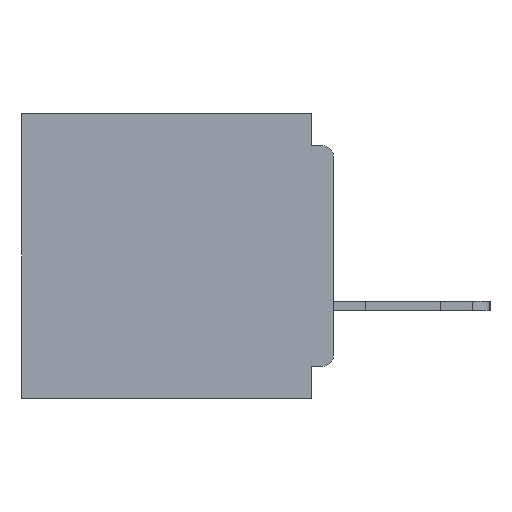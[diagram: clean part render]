
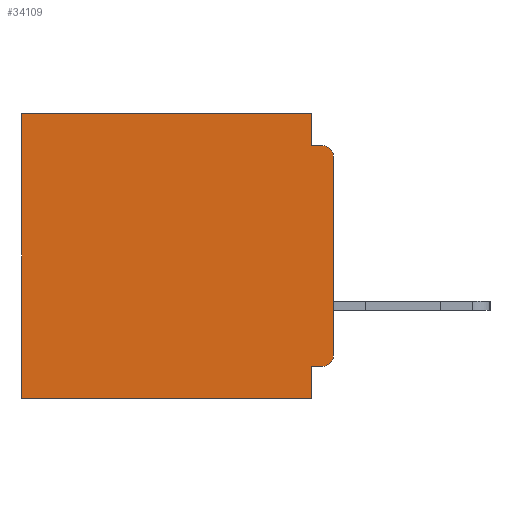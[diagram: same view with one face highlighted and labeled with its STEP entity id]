
A CAD part, left-side view. The second image highlights one B-rep face of the part: STEP entity #34109.
In plain terms, the highlighted planar face has unit normal (-1, 0, 0).
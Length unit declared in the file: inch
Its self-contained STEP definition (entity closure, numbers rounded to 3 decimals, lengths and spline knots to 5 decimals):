
#508 = EDGE_LOOP ( 'NONE', ( #7604, #32701, #13063, #24815, #25394, #37105, #4179, #37846, #33562, #59256 ) ) ;
#1082 = CARTESIAN_POINT ( 'NONE',  ( 0.3, 0., -0.4 ) ) ;
#1469 = VERTEX_POINT ( 'NONE', #15467 ) ;
#1531 = LINE ( 'NONE', #14332, #25078 ) ;
#3493 = CARTESIAN_POINT ( 'NONE',  ( 0.3, 0.015, -0.355 ) ) ;
#4179 = ORIENTED_EDGE ( 'NONE', *, *, #61066, .F. ) ;
#4317 = LINE ( 'NONE', #37463, #62940 ) ;
#5022 = DIRECTION ( 'NONE',  ( 0., 0., -1. ) ) ;
#5680 = EDGE_CURVE ( 'NONE', #12072, #39543, #38894, .T. ) ;
#5737 = CARTESIAN_POINT ( 'NONE',  ( 0.3, 0.031, -0.4 ) ) ;
#6200 = DIRECTION ( 'NONE',  ( 0., 0., -1. ) ) ;
#7165 = FACE_OUTER_BOUND ( 'NONE', #508, .T. ) ;
#7604 = ORIENTED_EDGE ( 'NONE', *, *, #63134, .F. ) ;
#8185 = LINE ( 'NONE', #50016, #62896 ) ;
#9714 = DIRECTION ( 'NONE',  ( -1., 0., 0. ) ) ;
#9831 = CARTESIAN_POINT ( 'NONE',  ( 0.3, 0., 0. ) ) ;
#12072 = VERTEX_POINT ( 'NONE', #62257 ) ;
#13063 = ORIENTED_EDGE ( 'NONE', *, *, #31377, .F. ) ;
#14090 = DIRECTION ( 'NONE',  ( 0., 0., -1. ) ) ;
#14332 = CARTESIAN_POINT ( 'NONE',  ( 0.3, 0., -0.4 ) ) ;
#14398 = AXIS2_PLACEMENT_3D ( 'NONE', #39656, #9714, #44661 ) ;
#14864 = DIRECTION ( 'NONE',  ( 0., 1., 0. ) ) ;
#15204 = VERTEX_POINT ( 'NONE', #45032 ) ;
#15467 = CARTESIAN_POINT ( 'NONE',  ( 0.3, 0., -0.06 ) ) ;
#15819 = LINE ( 'NONE', #63529, #40810 ) ;
#16685 = CARTESIAN_POINT ( 'NONE',  ( 0.3, 0.437, -0.4 ) ) ;
#16819 = DIRECTION ( 'NONE',  ( 0., 0., -1. ) ) ;
#17236 = VERTEX_POINT ( 'NONE', #46989 ) ;
#18697 = CARTESIAN_POINT ( 'NONE',  ( 0.3, 0.437, -0.4 ) ) ;
#19067 = LINE ( 'NONE', #9831, #30826 ) ;
#19278 = EDGE_CURVE ( 'NONE', #59796, #40644, #15819, .T. ) ;
#19718 = VERTEX_POINT ( 'NONE', #62181 ) ;
#19735 = VERTEX_POINT ( 'NONE', #27519 ) ;
#20062 = DIRECTION ( 'NONE',  ( 0., 0., -1. ) ) ;
#24815 = ORIENTED_EDGE ( 'NONE', *, *, #28228, .F. ) ;
#25078 = VECTOR ( 'NONE', #64109, 39.37008 ) ;
#25394 = ORIENTED_EDGE ( 'NONE', *, *, #55567, .T. ) ;
#25995 = VECTOR ( 'NONE', #14090, 39.37008 ) ;
#26359 = VERTEX_POINT ( 'NONE', #5737 ) ;
#27519 = CARTESIAN_POINT ( 'NONE',  ( 0.3, 0.031, 0. ) ) ;
#28228 = EDGE_CURVE ( 'NONE', #19735, #19718, #8185, .T. ) ;
#28792 = EDGE_CURVE ( 'NONE', #1469, #17236, #60868, .T. ) ;
#30826 = VECTOR ( 'NONE', #14864, 39.37008 ) ;
#31377 = EDGE_CURVE ( 'NONE', #19718, #17236, #4317, .T. ) ;
#32701 = ORIENTED_EDGE ( 'NONE', *, *, #28792, .T. ) ;
#33562 = ORIENTED_EDGE ( 'NONE', *, *, #19278, .F. ) ;
#33869 = EDGE_CURVE ( 'NONE', #40644, #26359, #36165, .T. ) ;
#34109 = ADVANCED_FACE ( 'NONE', ( #7165 ), #56031, .F. ) ;
#35050 = DIRECTION ( 'NONE',  ( -1., 0., 0. ) ) ;
#36165 = LINE ( 'NONE', #49058, #25995 ) ;
#36175 = DIRECTION ( 'NONE',  ( 1., 0., 0. ) ) ;
#37105 = ORIENTED_EDGE ( 'NONE', *, *, #5680, .T. ) ;
#37463 = CARTESIAN_POINT ( 'NONE',  ( 0.3, 0., -0.045 ) ) ;
#37846 = ORIENTED_EDGE ( 'NONE', *, *, #33869, .F. ) ;
#38677 = DIRECTION ( 'NONE',  ( 0., 1., 0. ) ) ;
#38894 = LINE ( 'NONE', #16685, #49047 ) ;
#39543 = VERTEX_POINT ( 'NONE', #18697 ) ;
#39656 = CARTESIAN_POINT ( 'NONE',  ( 0.3, 0.015, -0.06 ) ) ;
#40644 = VERTEX_POINT ( 'NONE', #55780 ) ;
#40810 = VECTOR ( 'NONE', #38677, 39.37008 ) ;
#43578 = CIRCLE ( 'NONE', #58782, 0.015 ) ;
#43614 = VECTOR ( 'NONE', #64041, 39.37008 ) ;
#43989 = CARTESIAN_POINT ( 'NONE',  ( 0.3, 0., -0.4 ) ) ;
#44661 = DIRECTION ( 'NONE',  ( 0., 0., -1. ) ) ;
#45032 = CARTESIAN_POINT ( 'NONE',  ( 0.3, 0., -0.34 ) ) ;
#46989 = CARTESIAN_POINT ( 'NONE',  ( 0.3, 0.015, -0.045 ) ) ;
#48586 = EDGE_CURVE ( 'NONE', #59796, #15204, #43578, .T. ) ;
#49047 = VECTOR ( 'NONE', #16819, 39.37008 ) ;
#49058 = CARTESIAN_POINT ( 'NONE',  ( 0.3, 0.031, -0.4 ) ) ;
#50016 = CARTESIAN_POINT ( 'NONE',  ( 0.3, 0.031, 0. ) ) ;
#51072 = AXIS2_PLACEMENT_3D ( 'NONE', #1082, #36175, #6200 ) ;
#55567 = EDGE_CURVE ( 'NONE', #19735, #12072, #19067, .T. ) ;
#55780 = CARTESIAN_POINT ( 'NONE',  ( 0.3, 0.031, -0.355 ) ) ;
#56031 = PLANE ( 'NONE',  #51072 ) ;
#58468 = LINE ( 'NONE', #43989, #43614 ) ;
#58782 = AXIS2_PLACEMENT_3D ( 'NONE', #63990, #35050, #5022 ) ;
#59256 = ORIENTED_EDGE ( 'NONE', *, *, #48586, .T. ) ;
#59796 = VERTEX_POINT ( 'NONE', #3493 ) ;
#60868 = CIRCLE ( 'NONE', #14398, 0.015 ) ;
#61066 = EDGE_CURVE ( 'NONE', #26359, #39543, #1531, .T. ) ;
#62181 = CARTESIAN_POINT ( 'NONE',  ( 0.3, 0.031, -0.045 ) ) ;
#62257 = CARTESIAN_POINT ( 'NONE',  ( 0.3, 0.437, 0. ) ) ;
#62324 = DIRECTION ( 'NONE',  ( 0., -1., 0. ) ) ;
#62896 = VECTOR ( 'NONE', #20062, 39.37008 ) ;
#62940 = VECTOR ( 'NONE', #62324, 39.37008 ) ;
#63134 = EDGE_CURVE ( 'NONE', #1469, #15204, #58468, .T. ) ;
#63529 = CARTESIAN_POINT ( 'NONE',  ( 0.3, 0., -0.355 ) ) ;
#63990 = CARTESIAN_POINT ( 'NONE',  ( 0.3, 0.015, -0.34 ) ) ;
#64041 = DIRECTION ( 'NONE',  ( 0., 0., -1. ) ) ;
#64109 = DIRECTION ( 'NONE',  ( 0., 1., 0. ) ) ;
